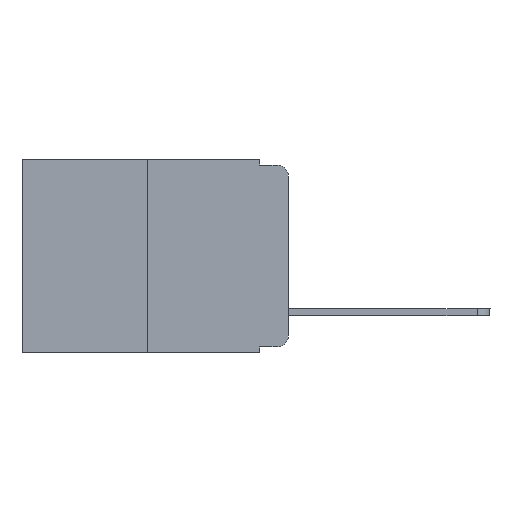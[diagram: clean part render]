
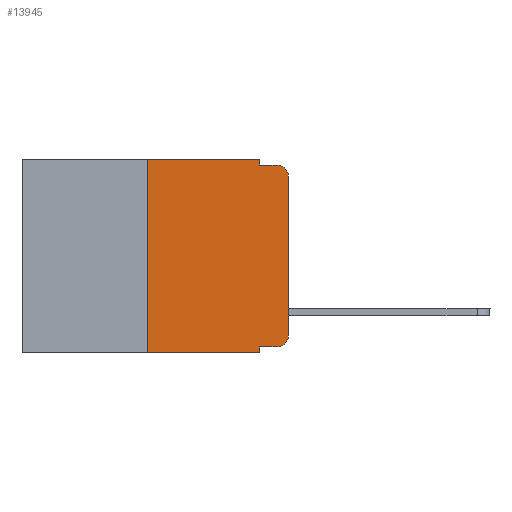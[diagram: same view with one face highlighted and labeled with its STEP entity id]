
A CAD part, left-side view. The second image highlights one B-rep face of the part: STEP entity #13945.
In plain terms, the highlighted planar face has unit normal (-1, 0, 0).
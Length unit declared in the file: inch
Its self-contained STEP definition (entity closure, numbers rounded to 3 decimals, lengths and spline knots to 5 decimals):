
#196 = VECTOR ( 'NONE', #10811, 39.37008 ) ;
#323 = CARTESIAN_POINT ( 'NONE',  ( 0., 0.25, 0. ) ) ;
#880 = VERTEX_POINT ( 'NONE', #4365 ) ;
#1097 = CARTESIAN_POINT ( 'NONE',  ( 0., 0.02, -0.333 ) ) ;
#1101 = VECTOR ( 'NONE', #14606, 39.37008 ) ;
#1162 = DIRECTION ( 'NONE',  ( -1., 0., 0. ) ) ;
#1238 = VECTOR ( 'NONE', #11173, 39.37008 ) ;
#1519 = CARTESIAN_POINT ( 'NONE',  ( 0., 0., 0. ) ) ;
#1558 = CARTESIAN_POINT ( 'NONE',  ( 0., 0.473, -0.343 ) ) ;
#1907 = VERTEX_POINT ( 'NONE', #4637 ) ;
#2021 = CARTESIAN_POINT ( 'NONE',  ( 0., 0.25, -0.343 ) ) ;
#2175 = VECTOR ( 'NONE', #4613, 39.37008 ) ;
#2413 = CARTESIAN_POINT ( 'NONE',  ( 0., 0., -0.313 ) ) ;
#2754 = DIRECTION ( 'NONE',  ( 0., 0., 1. ) ) ;
#2816 = CARTESIAN_POINT ( 'NONE',  ( 0., 0.051, -0.01 ) ) ;
#2926 = CARTESIAN_POINT ( 'NONE',  ( 0., 0., -0.03 ) ) ;
#3087 = EDGE_CURVE ( 'NONE', #10116, #1907, #15938, .T. ) ;
#3293 = EDGE_CURVE ( 'NONE', #10116, #6862, #4999, .T. ) ;
#3567 = DIRECTION ( 'NONE',  ( 0., -1., 0. ) ) ;
#3577 = EDGE_CURVE ( 'NONE', #6380, #12435, #5677, .T. ) ;
#3610 = CARTESIAN_POINT ( 'NONE',  ( 0., 0.25, 0. ) ) ;
#4015 = AXIS2_PLACEMENT_3D ( 'NONE', #6304, #8834, #15438 ) ;
#4032 = CIRCLE ( 'NONE', #11858, 0.02 ) ;
#4365 = CARTESIAN_POINT ( 'NONE',  ( 0., 0.02, -0.01 ) ) ;
#4404 = LINE ( 'NONE', #9673, #196 ) ;
#4613 = DIRECTION ( 'NONE',  ( 0., 0., 1. ) ) ;
#4637 = CARTESIAN_POINT ( 'NONE',  ( 0., 0.051, -0.343 ) ) ;
#4771 = EDGE_CURVE ( 'NONE', #13818, #880, #11127, .T. ) ;
#4999 = LINE ( 'NONE', #11465, #10827 ) ;
#5163 = ORIENTED_EDGE ( 'NONE', *, *, #10542, .F. ) ;
#5404 = VERTEX_POINT ( 'NONE', #2413 ) ;
#5677 = LINE ( 'NONE', #323, #2175 ) ;
#5768 = EDGE_CURVE ( 'NONE', #5404, #15822, #12208, .T. ) ;
#6050 = EDGE_CURVE ( 'NONE', #6862, #5404, #4032, .T. ) ;
#6304 = CARTESIAN_POINT ( 'NONE',  ( 0., 0.02, -0.03 ) ) ;
#6340 = ORIENTED_EDGE ( 'NONE', *, *, #3577, .F. ) ;
#6380 = VERTEX_POINT ( 'NONE', #2021 ) ;
#6474 = DIRECTION ( 'NONE',  ( 0., 0., -1. ) ) ;
#6539 = CARTESIAN_POINT ( 'NONE',  ( 0., 0.051, 0. ) ) ;
#6862 = VERTEX_POINT ( 'NONE', #1097 ) ;
#6902 = LINE ( 'NONE', #1558, #1238 ) ;
#7534 = DIRECTION ( 'NONE',  ( 0., -1., 0. ) ) ;
#7556 = ORIENTED_EDGE ( 'NONE', *, *, #16643, .T. ) ;
#7909 = ORIENTED_EDGE ( 'NONE', *, *, #6050, .T. ) ;
#8106 = VECTOR ( 'NONE', #3567, 39.37008 ) ;
#8834 = DIRECTION ( 'NONE',  ( -1., 0., 0. ) ) ;
#9018 = ORIENTED_EDGE ( 'NONE', *, *, #16419, .T. ) ;
#9240 = CARTESIAN_POINT ( 'NONE',  ( 0., 0.051, 0. ) ) ;
#9523 = CARTESIAN_POINT ( 'NONE',  ( 0., 0.051, -0.333 ) ) ;
#9673 = CARTESIAN_POINT ( 'NONE',  ( 0., 0.051, 0. ) ) ;
#10116 = VERTEX_POINT ( 'NONE', #9523 ) ;
#10252 = ORIENTED_EDGE ( 'NONE', *, *, #5768, .T. ) ;
#10405 = PLANE ( 'NONE',  #13443 ) ;
#10542 = EDGE_CURVE ( 'NONE', #15645, #13818, #4404, .T. ) ;
#10811 = DIRECTION ( 'NONE',  ( 0., 0., -1. ) ) ;
#10827 = VECTOR ( 'NONE', #7534, 39.37008 ) ;
#10900 = CARTESIAN_POINT ( 'NONE',  ( 0., 0.473, 0. ) ) ;
#11127 = LINE ( 'NONE', #2816, #13824 ) ;
#11173 = DIRECTION ( 'NONE',  ( 0., -1., 0. ) ) ;
#11465 = CARTESIAN_POINT ( 'NONE',  ( 0., 0.051, -0.333 ) ) ;
#11571 = EDGE_LOOP ( 'NONE', ( #10252, #9018, #15557, #5163, #13712, #6340, #7556, #15373, #15241, #7909 ) ) ;
#11858 = AXIS2_PLACEMENT_3D ( 'NONE', #13170, #1162, #13252 ) ;
#12208 = LINE ( 'NONE', #1519, #16648 ) ;
#12435 = VERTEX_POINT ( 'NONE', #3610 ) ;
#13170 = CARTESIAN_POINT ( 'NONE',  ( 0., 0.02, -0.313 ) ) ;
#13252 = DIRECTION ( 'NONE',  ( 0., 0., -1. ) ) ;
#13443 = AXIS2_PLACEMENT_3D ( 'NONE', #10900, #14631, #6474 ) ;
#13459 = EDGE_CURVE ( 'NONE', #12435, #15645, #15951, .T. ) ;
#13712 = ORIENTED_EDGE ( 'NONE', *, *, #13459, .F. ) ;
#13818 = VERTEX_POINT ( 'NONE', #15608 ) ;
#13824 = VECTOR ( 'NONE', #16503, 39.37008 ) ;
#13945 = ADVANCED_FACE ( 'NONE', ( #15786 ), #10405, .F. ) ;
#14606 = DIRECTION ( 'NONE',  ( 0., 0., -1. ) ) ;
#14631 = DIRECTION ( 'NONE',  ( 1., 0., 0. ) ) ;
#15241 = ORIENTED_EDGE ( 'NONE', *, *, #3293, .T. ) ;
#15373 = ORIENTED_EDGE ( 'NONE', *, *, #3087, .F. ) ;
#15438 = DIRECTION ( 'NONE',  ( 0., 0., -1. ) ) ;
#15557 = ORIENTED_EDGE ( 'NONE', *, *, #4771, .F. ) ;
#15597 = CARTESIAN_POINT ( 'NONE',  ( 0., 0.473, 0. ) ) ;
#15608 = CARTESIAN_POINT ( 'NONE',  ( 0., 0.051, -0.01 ) ) ;
#15645 = VERTEX_POINT ( 'NONE', #6539 ) ;
#15786 = FACE_OUTER_BOUND ( 'NONE', #11571, .T. ) ;
#15822 = VERTEX_POINT ( 'NONE', #2926 ) ;
#15938 = LINE ( 'NONE', #9240, #1101 ) ;
#15951 = LINE ( 'NONE', #15597, #8106 ) ;
#16419 = EDGE_CURVE ( 'NONE', #15822, #880, #16903, .T. ) ;
#16503 = DIRECTION ( 'NONE',  ( 0., -1., 0. ) ) ;
#16643 = EDGE_CURVE ( 'NONE', #6380, #1907, #6902, .T. ) ;
#16648 = VECTOR ( 'NONE', #2754, 39.37008 ) ;
#16903 = CIRCLE ( 'NONE', #4015, 0.02 ) ;
